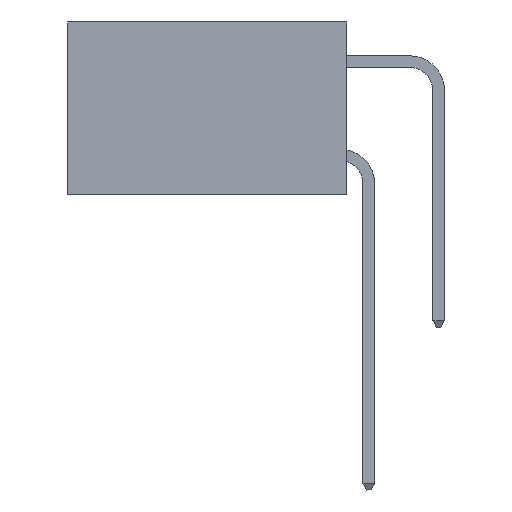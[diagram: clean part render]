
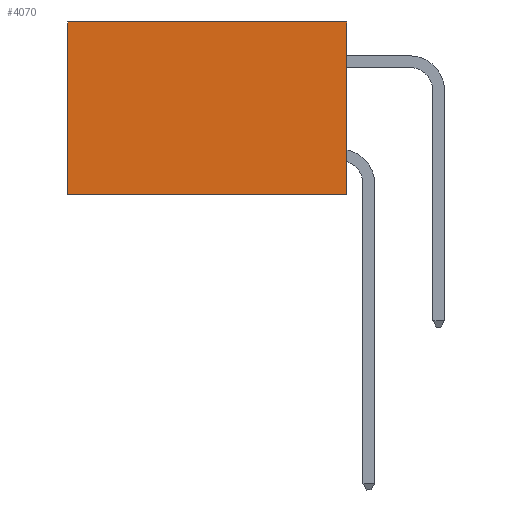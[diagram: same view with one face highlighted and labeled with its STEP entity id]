
A CAD part, left-side view. The second image highlights one B-rep face of the part: STEP entity #4070.
In plain terms, the highlighted planar face has unit normal (-1, 0, 0).
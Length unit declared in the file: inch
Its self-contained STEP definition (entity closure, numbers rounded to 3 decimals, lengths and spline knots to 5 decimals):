
#958 = DIRECTION ( 'NONE',  ( 1., 0., 0. ) ) ;
#1273 = DIRECTION ( 'NONE',  ( 0., 1., 0. ) ) ;
#1523 = ORIENTED_EDGE ( 'NONE', *, *, #12364, .T. ) ;
#2008 = LINE ( 'NONE', #14383, #19035 ) ;
#2901 = CARTESIAN_POINT ( 'NONE',  ( 0.2875, 0., 0. ) ) ;
#4070 = ADVANCED_FACE ( 'NONE', ( #13831 ), #5819, .F. ) ;
#5819 = PLANE ( 'NONE',  #10632 ) ;
#6768 = CARTESIAN_POINT ( 'NONE',  ( 0.2875, 0., -0.37 ) ) ;
#7246 = CARTESIAN_POINT ( 'NONE',  ( 0.2875, 0., 0. ) ) ;
#7407 = EDGE_CURVE ( 'NONE', #8426, #14980, #2008, .T. ) ;
#8165 = VECTOR ( 'NONE', #12767, 39.37008 ) ;
#8426 = VERTEX_POINT ( 'NONE', #6768 ) ;
#8717 = LINE ( 'NONE', #11544, #17019 ) ;
#8871 = ORIENTED_EDGE ( 'NONE', *, *, #16334, .F. ) ;
#10477 = CARTESIAN_POINT ( 'NONE',  ( 0.2875, 0., 0. ) ) ;
#10632 = AXIS2_PLACEMENT_3D ( 'NONE', #10761, #958, #12454 ) ;
#10761 = CARTESIAN_POINT ( 'NONE',  ( 0.2875, 0., 0. ) ) ;
#11418 = VERTEX_POINT ( 'NONE', #10477 ) ;
#11544 = CARTESIAN_POINT ( 'NONE',  ( 0.2875, 0.6, 0. ) ) ;
#12364 = EDGE_CURVE ( 'NONE', #12932, #14980, #8717, .T. ) ;
#12454 = DIRECTION ( 'NONE',  ( 0., 0., -1. ) ) ;
#12767 = DIRECTION ( 'NONE',  ( 0., 1., 0. ) ) ;
#12932 = VERTEX_POINT ( 'NONE', #14605 ) ;
#13247 = DIRECTION ( 'NONE',  ( 0., 0., -1. ) ) ;
#13831 = FACE_OUTER_BOUND ( 'NONE', #14914, .T. ) ;
#14383 = CARTESIAN_POINT ( 'NONE',  ( 0.2875, 0., -0.37 ) ) ;
#14605 = CARTESIAN_POINT ( 'NONE',  ( 0.2875, 0.6, 0. ) ) ;
#14914 = EDGE_LOOP ( 'NONE', ( #1523, #18275, #8871, #18583 ) ) ;
#14980 = VERTEX_POINT ( 'NONE', #17072 ) ;
#15977 = VECTOR ( 'NONE', #17156, 39.37008 ) ;
#16334 = EDGE_CURVE ( 'NONE', #11418, #8426, #20879, .T. ) ;
#17019 = VECTOR ( 'NONE', #13247, 39.37008 ) ;
#17072 = CARTESIAN_POINT ( 'NONE',  ( 0.2875, 0.6, -0.37 ) ) ;
#17156 = DIRECTION ( 'NONE',  ( 0., 0., -1. ) ) ;
#17884 = EDGE_CURVE ( 'NONE', #11418, #12932, #20040, .T. ) ;
#18275 = ORIENTED_EDGE ( 'NONE', *, *, #7407, .F. ) ;
#18583 = ORIENTED_EDGE ( 'NONE', *, *, #17884, .T. ) ;
#19035 = VECTOR ( 'NONE', #1273, 39.37008 ) ;
#20040 = LINE ( 'NONE', #2901, #8165 ) ;
#20879 = LINE ( 'NONE', #7246, #15977 ) ;
